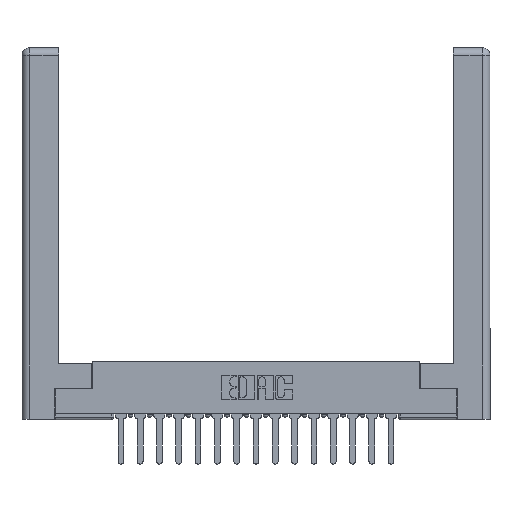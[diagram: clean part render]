
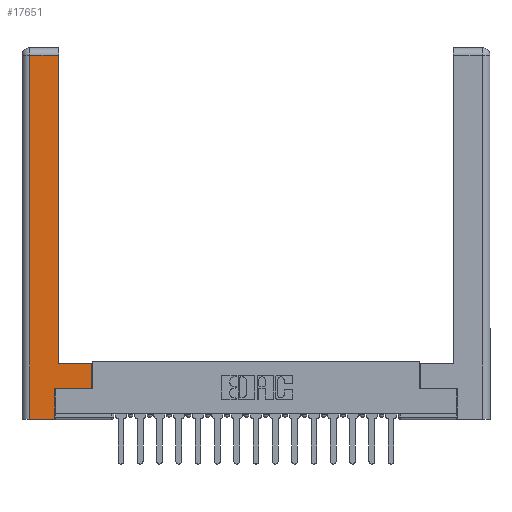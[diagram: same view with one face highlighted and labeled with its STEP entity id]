
A CAD part, top view. The second image highlights one B-rep face of the part: STEP entity #17651.
In plain terms, the highlighted planar face has unit normal (0, 0, 1).
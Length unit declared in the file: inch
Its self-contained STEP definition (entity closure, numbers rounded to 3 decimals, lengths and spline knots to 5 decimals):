
#259 = DIRECTION ( 'NONE',  ( 1., 0., 0. ) ) ;
#303 = PLANE ( 'NONE',  #6933 ) ;
#381 = VERTEX_POINT ( 'NONE', #4496 ) ;
#568 = EDGE_CURVE ( 'NONE', #7229, #381, #3827, .T. ) ;
#726 = VECTOR ( 'NONE', #14277, 39.37008 ) ;
#738 = EDGE_CURVE ( 'NONE', #6158, #11397, #18379, .T. ) ;
#1081 = ORIENTED_EDGE ( 'NONE', *, *, #18744, .T. ) ;
#1166 = LINE ( 'NONE', #7481, #4074 ) ;
#2231 = DIRECTION ( 'NONE',  ( 0., -1., 0. ) ) ;
#2317 = EDGE_LOOP ( 'NONE', ( #2679, #15663, #3840, #15567, #1081, #4367, #14799, #18398 ) ) ;
#2520 = CARTESIAN_POINT ( 'NONE',  ( 0.0615, 2.94, 0. ) ) ;
#2679 = ORIENTED_EDGE ( 'NONE', *, *, #568, .T. ) ;
#3222 = CARTESIAN_POINT ( 'NONE',  ( 0.295, 0.45, 0. ) ) ;
#3827 = LINE ( 'NONE', #13708, #7938 ) ;
#3840 = ORIENTED_EDGE ( 'NONE', *, *, #14639, .T. ) ;
#3957 = DIRECTION ( 'NONE',  ( 0., 0., -1. ) ) ;
#3960 = CARTESIAN_POINT ( 'NONE',  ( 0.265, 0.245, 0. ) ) ;
#4015 = CARTESIAN_POINT ( 'NONE',  ( 0.565, 0.245, 0. ) ) ;
#4074 = VECTOR ( 'NONE', #259, 39.37008 ) ;
#4367 = ORIENTED_EDGE ( 'NONE', *, *, #13944, .T. ) ;
#4496 = CARTESIAN_POINT ( 'NONE',  ( 0.295, 2.94, 0. ) ) ;
#4558 = EDGE_CURVE ( 'NONE', #13659, #7229, #15854, .T. ) ;
#4617 = CARTESIAN_POINT ( 'NONE',  ( 0.265, 0., 0. ) ) ;
#5073 = CARTESIAN_POINT ( 'NONE',  ( 0.0615, 0., 0. ) ) ;
#5464 = CARTESIAN_POINT ( 'NONE',  ( 0.0615, 0., 0. ) ) ;
#5606 = VECTOR ( 'NONE', #2231, 39.37008 ) ;
#6158 = VERTEX_POINT ( 'NONE', #5464 ) ;
#6379 = VECTOR ( 'NONE', #17066, 39.37008 ) ;
#6933 = AXIS2_PLACEMENT_3D ( 'NONE', #15555, #3957, #14207 ) ;
#7229 = VERTEX_POINT ( 'NONE', #3222 ) ;
#7465 = CARTESIAN_POINT ( 'NONE',  ( 0.565, 0.45, 0. ) ) ;
#7481 = CARTESIAN_POINT ( 'NONE',  ( 0.565, 0.245, 0. ) ) ;
#7564 = VECTOR ( 'NONE', #16984, 39.37008 ) ;
#7938 = VECTOR ( 'NONE', #12462, 39.37008 ) ;
#8302 = LINE ( 'NONE', #2520, #6379 ) ;
#8497 = EDGE_CURVE ( 'NONE', #381, #14065, #8302, .T. ) ;
#8507 = FACE_OUTER_BOUND ( 'NONE', #2317, .T. ) ;
#9465 = LINE ( 'NONE', #3960, #7564 ) ;
#10029 = EDGE_CURVE ( 'NONE', #13975, #13659, #10216, .T. ) ;
#10122 = CARTESIAN_POINT ( 'NONE',  ( 0.295, 0.45, 0. ) ) ;
#10216 = LINE ( 'NONE', #7465, #13695 ) ;
#10793 = CARTESIAN_POINT ( 'NONE',  ( 0.0615, 2.94, 0. ) ) ;
#11397 = VERTEX_POINT ( 'NONE', #4617 ) ;
#11643 = DIRECTION ( 'NONE',  ( -1., 0., 0. ) ) ;
#12462 = DIRECTION ( 'NONE',  ( 0., 1., 0. ) ) ;
#13659 = VERTEX_POINT ( 'NONE', #17616 ) ;
#13695 = VECTOR ( 'NONE', #14408, 39.37008 ) ;
#13708 = CARTESIAN_POINT ( 'NONE',  ( 0.295, 3., 0. ) ) ;
#13720 = LINE ( 'NONE', #5073, #5606 ) ;
#13944 = EDGE_CURVE ( 'NONE', #15413, #13975, #1166, .T. ) ;
#13975 = VERTEX_POINT ( 'NONE', #4015 ) ;
#14065 = VERTEX_POINT ( 'NONE', #10793 ) ;
#14207 = DIRECTION ( 'NONE',  ( -1., 0., 0. ) ) ;
#14277 = DIRECTION ( 'NONE',  ( 1., 0., 0. ) ) ;
#14408 = DIRECTION ( 'NONE',  ( 0., 1., 0. ) ) ;
#14639 = EDGE_CURVE ( 'NONE', #14065, #6158, #13720, .T. ) ;
#14799 = ORIENTED_EDGE ( 'NONE', *, *, #10029, .T. ) ;
#15413 = VERTEX_POINT ( 'NONE', #16175 ) ;
#15555 = CARTESIAN_POINT ( 'NONE',  ( 0., 0., 0. ) ) ;
#15567 = ORIENTED_EDGE ( 'NONE', *, *, #738, .T. ) ;
#15663 = ORIENTED_EDGE ( 'NONE', *, *, #8497, .T. ) ;
#15716 = CARTESIAN_POINT ( 'NONE',  ( 0.265, 0., 0. ) ) ;
#15854 = LINE ( 'NONE', #10122, #16659 ) ;
#16175 = CARTESIAN_POINT ( 'NONE',  ( 0.265, 0.245, 0. ) ) ;
#16659 = VECTOR ( 'NONE', #11643, 39.37008 ) ;
#16984 = DIRECTION ( 'NONE',  ( 0., 1., 0. ) ) ;
#17066 = DIRECTION ( 'NONE',  ( -1., 0., 0. ) ) ;
#17616 = CARTESIAN_POINT ( 'NONE',  ( 0.565, 0.45, 0. ) ) ;
#17651 = ADVANCED_FACE ( 'NONE', ( #8507 ), #303, .F. ) ;
#18379 = LINE ( 'NONE', #15716, #726 ) ;
#18398 = ORIENTED_EDGE ( 'NONE', *, *, #4558, .T. ) ;
#18744 = EDGE_CURVE ( 'NONE', #11397, #15413, #9465, .T. ) ;
